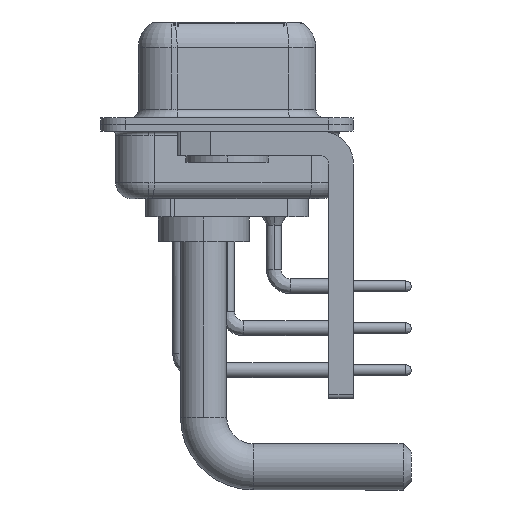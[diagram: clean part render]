
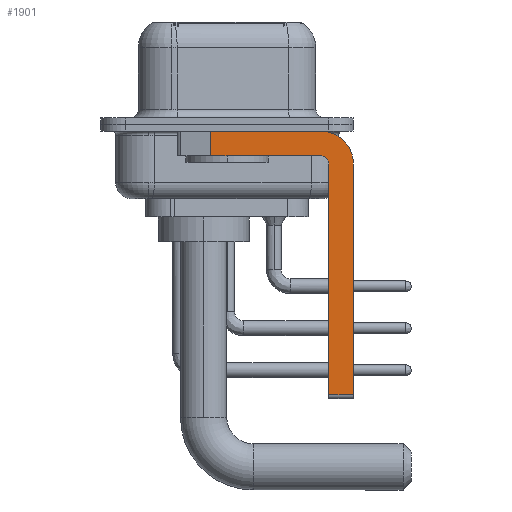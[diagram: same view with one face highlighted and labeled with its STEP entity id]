
A CAD part, left-side view. The second image highlights one B-rep face of the part: STEP entity #1901.
In plain terms, the highlighted planar face has unit normal (-1, 0, 0).
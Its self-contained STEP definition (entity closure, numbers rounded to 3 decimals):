
#1060 = AXIS2_PLACEMENT_3D ( 'NONE', #27379, #3943, #20241 ) ;
#1541 = ORIENTED_EDGE ( 'NONE', *, *, #21489, .F. ) ;
#1901 = ADVANCED_FACE ( 'NONE', ( #18114 ), #15665, .F. ) ;
#2192 = AXIS2_PLACEMENT_3D ( 'NONE', #5134, #14426, #23718 ) ;
#2503 = VECTOR ( 'NONE', #3179, 1000. ) ;
#2862 = EDGE_CURVE ( 'NONE', #3860, #8076, #6727, .T. ) ;
#3179 = DIRECTION ( 'NONE',  ( 0., 0., -1. ) ) ;
#3860 = VERTEX_POINT ( 'NONE', #19131 ) ;
#3943 = DIRECTION ( 'NONE',  ( 1., 0., 0. ) ) ;
#4492 = ORIENTED_EDGE ( 'NONE', *, *, #12837, .F. ) ;
#4625 = LINE ( 'NONE', #4915, #28937 ) ;
#4671 = EDGE_CURVE ( 'NONE', #3860, #13266, #15473, .T. ) ;
#4758 = CARTESIAN_POINT ( 'NONE',  ( -2.9, 0.978, -1.9 ) ) ;
#4915 = CARTESIAN_POINT ( 'NONE',  ( -2.9, -7.65, -2.4 ) ) ;
#5048 = ORIENTED_EDGE ( 'NONE', *, *, #13764, .F. ) ;
#5094 = CARTESIAN_POINT ( 'NONE',  ( -2.9, 0.978, -0.4 ) ) ;
#5134 = CARTESIAN_POINT ( 'NONE',  ( -2.9, -5.65, -2.4 ) ) ;
#6004 = DIRECTION ( 'NONE',  ( 0., 0., 1. ) ) ;
#6035 = CARTESIAN_POINT ( 'NONE',  ( -2.9, -5.65, -16.35 ) ) ;
#6727 = LINE ( 'NONE', #23311, #19654 ) ;
#6900 = CARTESIAN_POINT ( 'NONE',  ( -2.9, -5.65, -0.4 ) ) ;
#7634 = ORIENTED_EDGE ( 'NONE', *, *, #24343, .F. ) ;
#7908 = CARTESIAN_POINT ( 'NONE',  ( -2.9, -7.65, -16.35 ) ) ;
#8039 = CARTESIAN_POINT ( 'NONE',  ( -2.9, -5.65, -1.9 ) ) ;
#8044 = CARTESIAN_POINT ( 'NONE',  ( -2.9, 0.978, -1.9 ) ) ;
#8076 = VERTEX_POINT ( 'NONE', #12894 ) ;
#8292 = DIRECTION ( 'NONE',  ( -1., 0., 0. ) ) ;
#8950 = VECTOR ( 'NONE', #19545, 1000. ) ;
#9002 = VERTEX_POINT ( 'NONE', #24065 ) ;
#10372 = EDGE_CURVE ( 'NONE', #27077, #14980, #19895, .T. ) ;
#10723 = VECTOR ( 'NONE', #15166, 1000. ) ;
#10774 = CARTESIAN_POINT ( 'NONE',  ( -2.9, 3., -0.4 ) ) ;
#11432 = CIRCLE ( 'NONE', #2192, 2. ) ;
#11700 = VERTEX_POINT ( 'NONE', #8039 ) ;
#11794 = VECTOR ( 'NONE', #29185, 1000. ) ;
#12210 = ORIENTED_EDGE ( 'NONE', *, *, #4671, .T. ) ;
#12558 = CARTESIAN_POINT ( 'NONE',  ( -2.9, -5.65, -1.9 ) ) ;
#12597 = ORIENTED_EDGE ( 'NONE', *, *, #2862, .F. ) ;
#12837 = EDGE_CURVE ( 'NONE', #11700, #27557, #29131, .T. ) ;
#12894 = CARTESIAN_POINT ( 'NONE',  ( -2.9, -6.15, -2.4 ) ) ;
#13266 = VERTEX_POINT ( 'NONE', #7908 ) ;
#13764 = EDGE_CURVE ( 'NONE', #14980, #9002, #11432, .T. ) ;
#13777 = AXIS2_PLACEMENT_3D ( 'NONE', #29142, #8292, #6004 ) ;
#14426 = DIRECTION ( 'NONE',  ( 1., 0., 0. ) ) ;
#14980 = VERTEX_POINT ( 'NONE', #6900 ) ;
#15166 = DIRECTION ( 'NONE',  ( 0., -1., 0. ) ) ;
#15473 = LINE ( 'NONE', #6035, #10723 ) ;
#15665 = PLANE ( 'NONE',  #1060 ) ;
#15849 = EDGE_LOOP ( 'NONE', ( #17930, #19067, #4492, #1541, #12597, #12210, #7634, #5048 ) ) ;
#17930 = ORIENTED_EDGE ( 'NONE', *, *, #10372, .F. ) ;
#18114 = FACE_OUTER_BOUND ( 'NONE', #15849, .T. ) ;
#19067 = ORIENTED_EDGE ( 'NONE', *, *, #28599, .T. ) ;
#19131 = CARTESIAN_POINT ( 'NONE',  ( -2.9, -6.15, -16.35 ) ) ;
#19545 = DIRECTION ( 'NONE',  ( 0., 1., 0. ) ) ;
#19654 = VECTOR ( 'NONE', #20428, 1000. ) ;
#19895 = LINE ( 'NONE', #10774, #11794 ) ;
#20241 = DIRECTION ( 'NONE',  ( 0., 0., -1. ) ) ;
#20428 = DIRECTION ( 'NONE',  ( 0., 0., 1. ) ) ;
#21489 = EDGE_CURVE ( 'NONE', #8076, #11700, #24001, .T. ) ;
#23311 = CARTESIAN_POINT ( 'NONE',  ( -2.9, -6.15, -16.6 ) ) ;
#23718 = DIRECTION ( 'NONE',  ( 0., 0., -1. ) ) ;
#24001 = CIRCLE ( 'NONE', #13777, 0.5 ) ;
#24065 = CARTESIAN_POINT ( 'NONE',  ( -2.9, -7.65, -2.4 ) ) ;
#24340 = LINE ( 'NONE', #8044, #2503 ) ;
#24343 = EDGE_CURVE ( 'NONE', #9002, #13266, #4625, .T. ) ;
#27077 = VERTEX_POINT ( 'NONE', #5094 ) ;
#27379 = CARTESIAN_POINT ( 'NONE',  ( -2.9, -5.65, -2.4 ) ) ;
#27466 = DIRECTION ( 'NONE',  ( 0., 0., -1. ) ) ;
#27557 = VERTEX_POINT ( 'NONE', #4758 ) ;
#28599 = EDGE_CURVE ( 'NONE', #27077, #27557, #24340, .T. ) ;
#28937 = VECTOR ( 'NONE', #27466, 1000. ) ;
#29131 = LINE ( 'NONE', #12558, #8950 ) ;
#29142 = CARTESIAN_POINT ( 'NONE',  ( -2.9, -5.65, -2.4 ) ) ;
#29185 = DIRECTION ( 'NONE',  ( 0., -1., 0. ) ) ;
